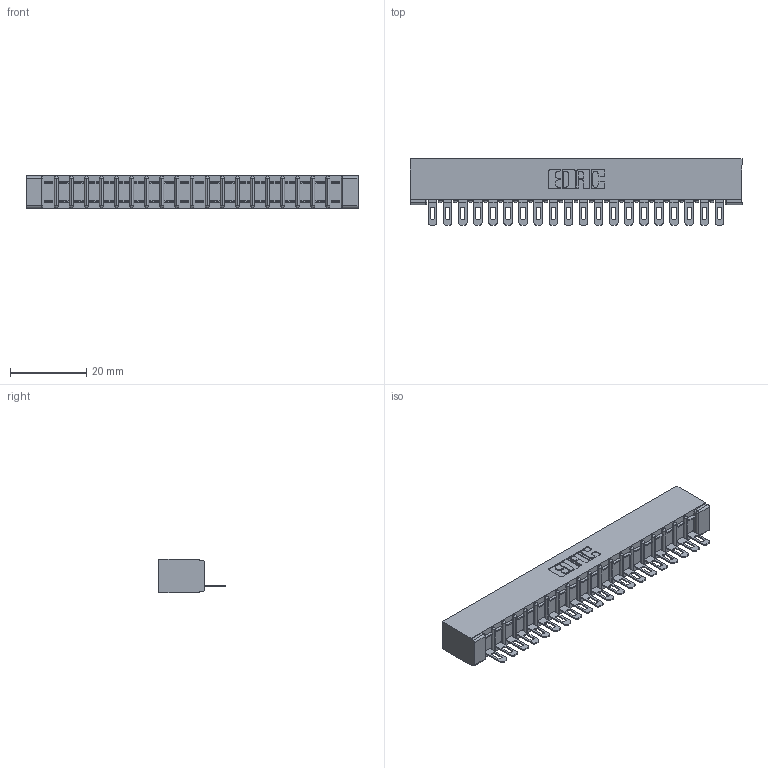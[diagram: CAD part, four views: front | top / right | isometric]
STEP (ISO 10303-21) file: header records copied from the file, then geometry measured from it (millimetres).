
FILE_DESCRIPTION (( 'STEP AP203' ), '1' );
FILE_NAME ('307-020-501-101.STEP', '2019-09-04T22:55:28', ( '' ), ( '' ), 'SwSTEP 2.0', 'SolidWorks 2016', '' );
FILE_SCHEMA (( 'CONFIG_CONTROL_DESIGN' ));
Length unit declared in the file: inch
Products named in the file (3): 307-290-002_501; 307-020-501-101; 307 Part_No Mounting Lugs
Assembly tree (21 placements, depth 2):
  307-020-501-101
    307 Part_No Mounting Lugs
    307-290-002_501  x20
Bounding box: 87.12 x 17.42 x 8.71 mm (x, y, z)
Volume: 6010.3 mm3; surface area: 11462.4 mm2
Topology: 21 solids, 21 shells, 1651 faces, 5059 edges, 3314 vertices
Faces by surface type: plane 946, cylinder 663, sphere 42
Entity records: 20374 total; most frequent: CARTESIAN_POINT 3432, ORIENTED_EDGE 3422, DIRECTION 3347, EDGE_CURVE 1711, VECTOR 1297, LINE 1297, VERTEX_POINT 1110, AXIS2_PLACEMENT_3D 1025
